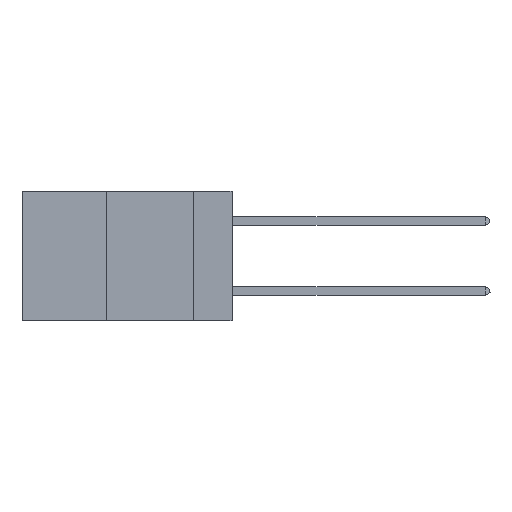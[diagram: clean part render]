
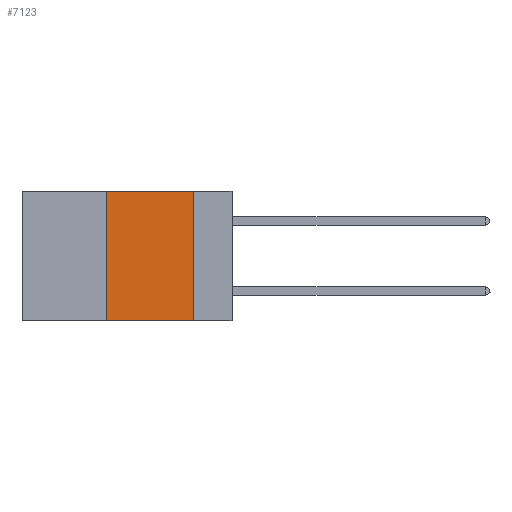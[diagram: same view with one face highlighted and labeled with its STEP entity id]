
A CAD part, left-side view. The second image highlights one B-rep face of the part: STEP entity #7123.
In plain terms, the highlighted planar face has unit normal (-1, 0, 0).
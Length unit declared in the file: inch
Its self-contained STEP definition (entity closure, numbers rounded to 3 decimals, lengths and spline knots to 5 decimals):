
#487 = DIRECTION ( 'NONE',  ( 1., 0., 0. ) ) ;
#2169 = VECTOR ( 'NONE', #24557, 39.37008 ) ;
#2526 = AXIS2_PLACEMENT_3D ( 'NONE', #7033, #487, #26049 ) ;
#2637 = DIRECTION ( 'NONE',  ( 0., -1., 0. ) ) ;
#2697 = PLANE ( 'NONE',  #2526 ) ;
#3133 = CARTESIAN_POINT ( 'NONE',  ( 0., 0.6, -0.37 ) ) ;
#3633 = EDGE_CURVE ( 'NONE', #23677, #7888, #9240, .T. ) ;
#4365 = LINE ( 'NONE', #16052, #14252 ) ;
#4967 = EDGE_CURVE ( 'NONE', #18461, #7888, #12470, .T. ) ;
#5547 = DIRECTION ( 'NONE',  ( 0., 0., 1. ) ) ;
#7033 = CARTESIAN_POINT ( 'NONE',  ( 0., 0.6, 0. ) ) ;
#7123 = ADVANCED_FACE ( 'NONE', ( #22687 ), #2697, .F. ) ;
#7542 = VECTOR ( 'NONE', #2637, 39.37008 ) ;
#7888 = VERTEX_POINT ( 'NONE', #17582 ) ;
#7966 = VECTOR ( 'NONE', #9212, 39.37008 ) ;
#9113 = ORIENTED_EDGE ( 'NONE', *, *, #4967, .T. ) ;
#9212 = DIRECTION ( 'NONE',  ( 0., 0., -1. ) ) ;
#9240 = LINE ( 'NONE', #24229, #7966 ) ;
#11953 = VERTEX_POINT ( 'NONE', #23447 ) ;
#12336 = EDGE_LOOP ( 'NONE', ( #16350, #21061, #25930, #9113 ) ) ;
#12470 = LINE ( 'NONE', #3133, #7542 ) ;
#14252 = VECTOR ( 'NONE', #5547, 39.37008 ) ;
#14361 = EDGE_CURVE ( 'NONE', #11953, #23677, #20563, .T. ) ;
#16052 = CARTESIAN_POINT ( 'NONE',  ( 0., 0.36, 0. ) ) ;
#16350 = ORIENTED_EDGE ( 'NONE', *, *, #3633, .F. ) ;
#16496 = EDGE_CURVE ( 'NONE', #18461, #11953, #4365, .T. ) ;
#17582 = CARTESIAN_POINT ( 'NONE',  ( 0., 0.11, -0.37 ) ) ;
#18305 = CARTESIAN_POINT ( 'NONE',  ( 0., 0.11, 0. ) ) ;
#18461 = VERTEX_POINT ( 'NONE', #26323 ) ;
#19518 = CARTESIAN_POINT ( 'NONE',  ( 0., 0.6, 0. ) ) ;
#20563 = LINE ( 'NONE', #19518, #2169 ) ;
#21061 = ORIENTED_EDGE ( 'NONE', *, *, #14361, .F. ) ;
#22687 = FACE_OUTER_BOUND ( 'NONE', #12336, .T. ) ;
#23447 = CARTESIAN_POINT ( 'NONE',  ( 0., 0.36, 0. ) ) ;
#23677 = VERTEX_POINT ( 'NONE', #18305 ) ;
#24229 = CARTESIAN_POINT ( 'NONE',  ( 0., 0.11, 0. ) ) ;
#24557 = DIRECTION ( 'NONE',  ( 0., -1., 0. ) ) ;
#25930 = ORIENTED_EDGE ( 'NONE', *, *, #16496, .F. ) ;
#26049 = DIRECTION ( 'NONE',  ( 0., 0., -1. ) ) ;
#26323 = CARTESIAN_POINT ( 'NONE',  ( 0., 0.36, -0.37 ) ) ;
